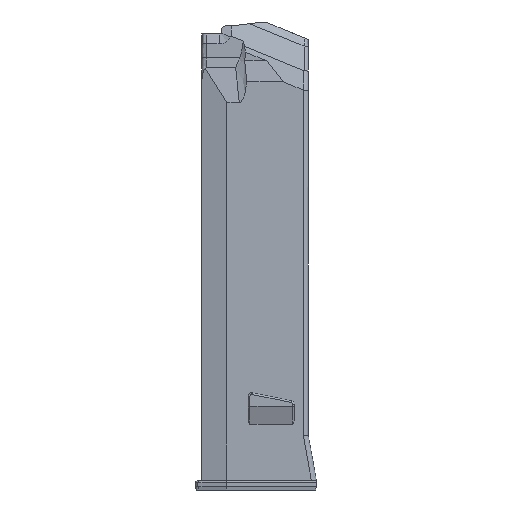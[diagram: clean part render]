
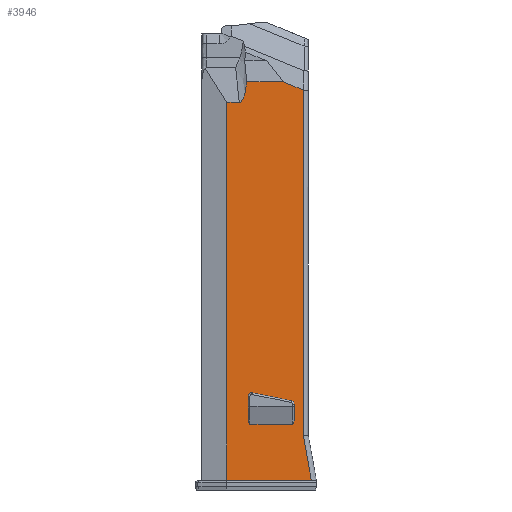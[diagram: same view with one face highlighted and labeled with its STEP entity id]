
A CAD part, left-side view. The second image highlights one B-rep face of the part: STEP entity #3946.
In plain terms, the highlighted planar face has unit normal (-1, 0, 0).
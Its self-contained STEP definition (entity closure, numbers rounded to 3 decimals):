
#184=FACE_BOUND('',#619,.T.);
#239=ELLIPSE('',#4232,1.463,0.503);
#240=ELLIPSE('',#4233,1.005,1.);
#241=ELLIPSE('',#4234,1.005,1.);
#242=ELLIPSE('',#4235,1.463,0.503);
#384=FACE_OUTER_BOUND('',#618,.T.);
#618=EDGE_LOOP('',(#2921,#2922,#2923,#2924,#2925,#2926,#2927,#2928));
#619=EDGE_LOOP('',(#2929,#2930,#2931,#2932,#2933,#2934,#2935,#2936));
#818=B_SPLINE_CURVE_WITH_KNOTS('',3,(#6410,#6411,#6412,#6413,#6414,#6415,
#6416,#6417,#6418,#6419,#6420,#6421,#6422),.UNSPECIFIED.,.F.,.F.,(4,3,3,
3,4),(0.44,0.612,0.907,1.091,
1.202),.UNSPECIFIED.);
#943=LINE('',#5247,#1252);
#947=LINE('',#5283,#1256);
#953=LINE('',#5306,#1262);
#1085=LINE('',#6246,#1394);
#1098=LINE('',#6423,#1407);
#1099=LINE('',#6425,#1408);
#1100=LINE('',#6426,#1409);
#1101=LINE('',#6429,#1410);
#1102=LINE('',#6433,#1411);
#1103=LINE('',#6437,#1412);
#1104=LINE('',#6441,#1413);
#1252=VECTOR('',#4398,10.);
#1256=VECTOR('',#4406,10.);
#1262=VECTOR('',#4418,10.043);
#1394=VECTOR('',#4724,10.05);
#1407=VECTOR('',#4767,10.05);
#1408=VECTOR('',#4768,10.002);
#1409=VECTOR('',#4769,10.);
#1410=VECTOR('',#4770,10.05);
#1411=VECTOR('',#4773,10.);
#1412=VECTOR('',#4776,10.048);
#1413=VECTOR('',#4779,10.);
#1561=VERTEX_POINT('',#5244);
#1562=VERTEX_POINT('',#5246);
#1567=VERTEX_POINT('',#5277);
#1568=VERTEX_POINT('',#5282);
#1574=VERTEX_POINT('',#5305);
#1709=VERTEX_POINT('',#6244);
#1731=VERTEX_POINT('',#6409);
#1732=VERTEX_POINT('',#6424);
#1733=VERTEX_POINT('',#6427);
#1734=VERTEX_POINT('',#6428);
#1735=VERTEX_POINT('',#6430);
#1736=VERTEX_POINT('',#6432);
#1737=VERTEX_POINT('',#6434);
#1738=VERTEX_POINT('',#6436);
#1739=VERTEX_POINT('',#6438);
#1740=VERTEX_POINT('',#6440);
#1945=EDGE_CURVE('',#1562,#1561,#943,.T.);
#1952=EDGE_CURVE('',#1568,#1567,#947,.T.);
#1960=EDGE_CURVE('',#1568,#1574,#953,.T.);
#2153=EDGE_CURVE('',#1709,#1561,#1085,.T.);
#2185=EDGE_CURVE('',#1731,#1567,#818,.F.);
#2186=EDGE_CURVE('',#1562,#1731,#1098,.T.);
#2187=EDGE_CURVE('',#1732,#1709,#1099,.T.);
#2188=EDGE_CURVE('',#1574,#1732,#1100,.T.);
#2189=EDGE_CURVE('',#1733,#1734,#1101,.T.);
#2190=EDGE_CURVE('',#1733,#1735,#239,.F.);
#2191=EDGE_CURVE('',#1736,#1735,#1102,.T.);
#2192=EDGE_CURVE('',#1736,#1737,#240,.F.);
#2193=EDGE_CURVE('',#1738,#1737,#1103,.T.);
#2194=EDGE_CURVE('',#1738,#1739,#241,.F.);
#2195=EDGE_CURVE('',#1740,#1739,#1104,.T.);
#2196=EDGE_CURVE('',#1740,#1734,#242,.F.);
#2921=ORIENTED_EDGE('',*,*,#1952,.T.);
#2922=ORIENTED_EDGE('',*,*,#2185,.F.);
#2923=ORIENTED_EDGE('',*,*,#2186,.F.);
#2924=ORIENTED_EDGE('',*,*,#1945,.T.);
#2925=ORIENTED_EDGE('',*,*,#2153,.F.);
#2926=ORIENTED_EDGE('',*,*,#2187,.F.);
#2927=ORIENTED_EDGE('',*,*,#2188,.F.);
#2928=ORIENTED_EDGE('',*,*,#1960,.F.);
#2929=ORIENTED_EDGE('',*,*,#2189,.F.);
#2930=ORIENTED_EDGE('',*,*,#2190,.T.);
#2931=ORIENTED_EDGE('',*,*,#2191,.F.);
#2932=ORIENTED_EDGE('',*,*,#2192,.T.);
#2933=ORIENTED_EDGE('',*,*,#2193,.F.);
#2934=ORIENTED_EDGE('',*,*,#2194,.T.);
#2935=ORIENTED_EDGE('',*,*,#2195,.F.);
#2936=ORIENTED_EDGE('',*,*,#2196,.T.);
#3824=PLANE('',#4231);
#3946=ADVANCED_FACE('',(#384,#184),#3824,.T.);
#4231=AXIS2_PLACEMENT_3D('',#6408,#4765,#4766);
#4232=AXIS2_PLACEMENT_3D('',#6431,#4771,#4772);
#4233=AXIS2_PLACEMENT_3D('',#6435,#4774,#4775);
#4234=AXIS2_PLACEMENT_3D('',#6439,#4777,#4778);
#4235=AXIS2_PLACEMENT_3D('',#6442,#4780,#4781);
#4398=DIRECTION('',(0.,0.,-1.));
#4406=DIRECTION('',(0.,1.,0.));
#4418=DIRECTION('',(0.,-0.925,-0.381));
#4724=DIRECTION('',(0.,1.,0.));
#4765=DIRECTION('center_axis',(-1.,0.,0.));
#4766=DIRECTION('ref_axis',(0.,0.,1.));
#4767=DIRECTION('',(0.,-1.,0.));
#4768=DIRECTION('',(0.,-0.177,-0.984));
#4769=DIRECTION('',(0.,0.,-1.));
#4770=DIRECTION('',(0.,-1.,0.));
#4771=DIRECTION('center_axis',(-1.,0.,0.));
#4772=DIRECTION('ref_axis',(0.,0.,
-1.));
#4773=DIRECTION('',(0.,0.,-1.));
#4774=DIRECTION('center_axis',(-1.,0.,0.));
#4775=DIRECTION('ref_axis',(0.,1.,0.));
#4776=DIRECTION('',(0.,0.98,0.198));
#4777=DIRECTION('center_axis',(-1.,0.,0.));
#4778=DIRECTION('ref_axis',(0.,1.,0.));
#4779=DIRECTION('',(0.,0.,1.));
#4780=DIRECTION('center_axis',(-1.,0.,0.));
#4781=DIRECTION('ref_axis',(0.,0.,-1.));
#5244=CARTESIAN_POINT('',(-10.509,8.562,3.05));
#5246=CARTESIAN_POINT('',(-10.509,8.562,118.95));
#5247=CARTESIAN_POINT('',(-10.509,8.562,6.3));
#5277=CARTESIAN_POINT('',(-10.509,2.449,125.254));
#5282=CARTESIAN_POINT('',(-10.509,-8.781,125.254));
#5283=CARTESIAN_POINT('',(-10.509,-5.828,125.254));
#5305=CARTESIAN_POINT('',(-10.509,-14.905,122.73));
#5306=CARTESIAN_POINT('',(-10.509,-32.689,115.4));
#6244=CARTESIAN_POINT('',(-10.509,-17.349,3.05));
#6246=CARTESIAN_POINT('',(-10.509,-8.253,3.05));
#6408=CARTESIAN_POINT('Origin',(-10.509,-16.413,6.3));
#6409=CARTESIAN_POINT('',(-10.509,4.756,118.95));
#6410=CARTESIAN_POINT('Ctrl Pts',(-10.509,2.449,125.254));
#6411=CARTESIAN_POINT('Ctrl Pts',(-10.509,2.513,124.671));
#6412=CARTESIAN_POINT('Ctrl Pts',(-10.509,2.587,124.084));
#6413=CARTESIAN_POINT('Ctrl Pts',(-10.509,2.683,123.473));
#6414=CARTESIAN_POINT('Ctrl Pts',(-10.509,2.847,122.43));
#6415=CARTESIAN_POINT('Ctrl Pts',(-10.509,3.069,121.378));
#6416=CARTESIAN_POINT('Ctrl Pts',(-10.509,3.372,120.551));
#6417=CARTESIAN_POINT('Ctrl Pts',(-10.509,3.561,120.035));
#6418=CARTESIAN_POINT('Ctrl Pts',(-10.509,3.77,119.598));
#6419=CARTESIAN_POINT('Ctrl Pts',(-10.509,4.077,119.28));
#6420=CARTESIAN_POINT('Ctrl Pts',(-10.509,4.262,119.089));
#6421=CARTESIAN_POINT('Ctrl Pts',(-10.509,4.496,118.95));
#6422=CARTESIAN_POINT('Ctrl Pts',(-10.509,4.756,118.95));
#6423=CARTESIAN_POINT('',(-10.509,-0.081,118.95));
#6424=CARTESIAN_POINT('',(-10.509,-14.905,16.667));
#6425=CARTESIAN_POINT('',(-10.509,-16.47,7.949));
#6426=CARTESIAN_POINT('',(-10.509,-14.905,6.3));
#6427=CARTESIAN_POINT('',(-10.509,1.494,20.2));
#6428=CARTESIAN_POINT('',(-10.509,-11.571,20.2));
#6429=CARTESIAN_POINT('',(-10.509,-14.243,20.2));
#6430=CARTESIAN_POINT('',(-10.509,1.997,21.663));
#6431=CARTESIAN_POINT('Origin',(-10.509,1.494,21.663));
#6432=CARTESIAN_POINT('',(-10.509,1.997,28.824));
#6433=CARTESIAN_POINT('',(-10.509,1.997,13.25));
#6434=CARTESIAN_POINT('',(-10.509,0.792,29.804));
#6435=CARTESIAN_POINT('Origin',(-10.509,0.992,28.824));
#6436=CARTESIAN_POINT('',(-10.509,-11.268,27.363));
#6437=CARTESIAN_POINT('',(-10.509,-9.173,27.787));
#6438=CARTESIAN_POINT('',(-10.509,-12.073,26.383));
#6439=CARTESIAN_POINT('Origin',(-10.509,-11.068,26.383));
#6440=CARTESIAN_POINT('',(-10.509,-12.073,21.663));
#6441=CARTESIAN_POINT('',(-10.509,-12.073,16.75));
#6442=CARTESIAN_POINT('Origin',(-10.509,-11.571,21.663));
